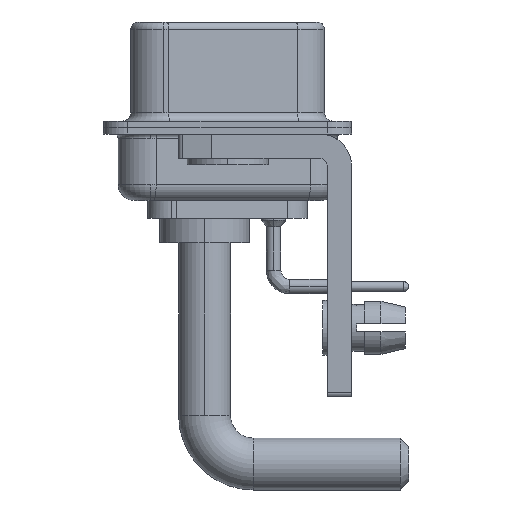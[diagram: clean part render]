
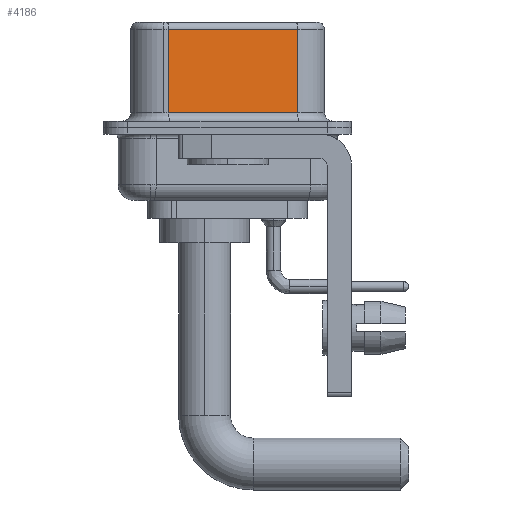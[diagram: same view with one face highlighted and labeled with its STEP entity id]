
A CAD part, left-side view. The second image highlights one B-rep face of the part: STEP entity #4186.
In plain terms, the highlighted planar face has unit normal (-0.985, -0.174, 0).
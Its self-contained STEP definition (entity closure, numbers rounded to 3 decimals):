
#1124 = VECTOR ( 'NONE', #22568, 1000. ) ;
#1391 = LINE ( 'NONE', #25845, #9801 ) ;
#2368 = LINE ( 'NONE', #12305, #15593 ) ;
#3285 = CARTESIAN_POINT ( 'NONE',  ( 5.132, -4.322, 6.52 ) ) ;
#3467 = VERTEX_POINT ( 'NONE', #17218 ) ;
#4186 = ADVANCED_FACE ( 'NONE', ( #11720 ), #26102, .F. ) ;
#5267 = ORIENTED_EDGE ( 'NONE', *, *, #17363, .T. ) ;
#5276 = LINE ( 'NONE', #3285, #15613 ) ;
#5752 = CARTESIAN_POINT ( 'NONE',  ( 5.132, -4.322, 6.02 ) ) ;
#6240 = EDGE_CURVE ( 'NONE', #25621, #18195, #2368, .T. ) ;
#6807 = EDGE_LOOP ( 'NONE', ( #14278, #16842, #5267, #14539 ) ) ;
#7005 = EDGE_CURVE ( 'NONE', #3467, #13631, #1391, .T. ) ;
#9748 = AXIS2_PLACEMENT_3D ( 'NONE', #9868, #21716, #11603 ) ;
#9801 = VECTOR ( 'NONE', #15584, 1000. ) ;
#9868 = CARTESIAN_POINT ( 'NONE',  ( 5.132, -4.322, 6.52 ) ) ;
#11603 = DIRECTION ( 'NONE',  ( -0.174, 0.985, 0. ) ) ;
#11720 = FACE_OUTER_BOUND ( 'NONE', #6807, .T. ) ;
#12174 = DIRECTION ( 'NONE',  ( -0.174, 0.985, 0. ) ) ;
#12305 = CARTESIAN_POINT ( 'NONE',  ( 5.132, -4.322, 6.02 ) ) ;
#13249 = CARTESIAN_POINT ( 'NONE',  ( 5.132, -4.322, 0.9 ) ) ;
#13631 = VERTEX_POINT ( 'NONE', #13249 ) ;
#14278 = ORIENTED_EDGE ( 'NONE', *, *, #18886, .F. ) ;
#14539 = ORIENTED_EDGE ( 'NONE', *, *, #7005, .T. ) ;
#14597 = CARTESIAN_POINT ( 'NONE',  ( 3.73, 3.628, 6.02 ) ) ;
#15584 = DIRECTION ( 'NONE',  ( 0.174, -0.985, 0. ) ) ;
#15593 = VECTOR ( 'NONE', #12174, 1000. ) ;
#15613 = VECTOR ( 'NONE', #17975, 1000. ) ;
#16842 = ORIENTED_EDGE ( 'NONE', *, *, #6240, .T. ) ;
#17218 = CARTESIAN_POINT ( 'NONE',  ( 3.73, 3.628, 0.9 ) ) ;
#17363 = EDGE_CURVE ( 'NONE', #18195, #3467, #22299, .T. ) ;
#17975 = DIRECTION ( 'NONE',  ( 0., 0., -1. ) ) ;
#18161 = CARTESIAN_POINT ( 'NONE',  ( 3.73, 3.628, 6.52 ) ) ;
#18195 = VERTEX_POINT ( 'NONE', #14597 ) ;
#18886 = EDGE_CURVE ( 'NONE', #25621, #13631, #5276, .T. ) ;
#21716 = DIRECTION ( 'NONE',  ( 0.985, 0.174, 0. ) ) ;
#22299 = LINE ( 'NONE', #18161, #1124 ) ;
#22568 = DIRECTION ( 'NONE',  ( 0., 0., -1. ) ) ;
#25621 = VERTEX_POINT ( 'NONE', #5752 ) ;
#25845 = CARTESIAN_POINT ( 'NONE',  ( 5.132, -4.322, 0.9 ) ) ;
#26102 = PLANE ( 'NONE',  #9748 ) ;
